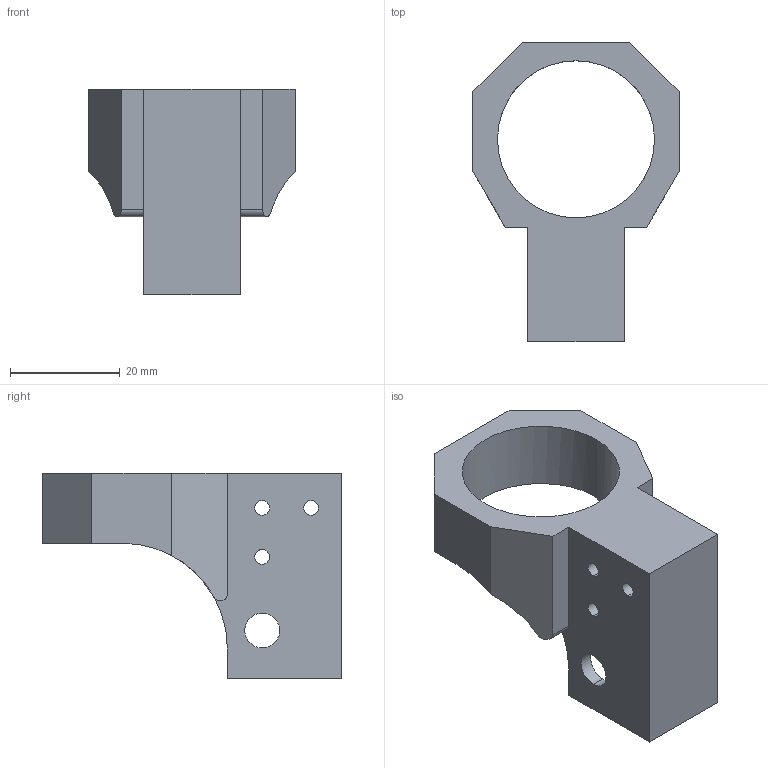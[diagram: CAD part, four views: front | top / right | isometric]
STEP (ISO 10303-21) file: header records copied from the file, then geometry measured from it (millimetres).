
FILE_DESCRIPTION (( 'STEP AP214' ), '1' );
FILE_NAME ('Original_Buffer.step', '2015-06-12T14:16:49', ( '' ), ( '' ), 'SwSTEP 2.0', 'SolidWorks 2015', '' );
FILE_SCHEMA (( 'AUTOMOTIVE_DESIGN' ));
Length unit declared in the file: inch
Products named in the file (1): Original_Buffer
Bounding box: 37.49 x 54.46 x 37.47 mm (x, y, z)
Volume: 17343.1 mm3; surface area: 8237.5 mm2
Topology: 1 solids, 1 shells, 44 faces, 132 edges, 88 vertices
Faces by surface type: plane 23, cylinder 21
Entity records: 1696 total; most frequent: CARTESIAN_POINT 435, ORIENTED_EDGE 264, DIRECTION 246, EDGE_CURVE 132, VERTEX_POINT 88, AXIS2_PLACEMENT_3D 85, VECTOR 76, LINE 76
